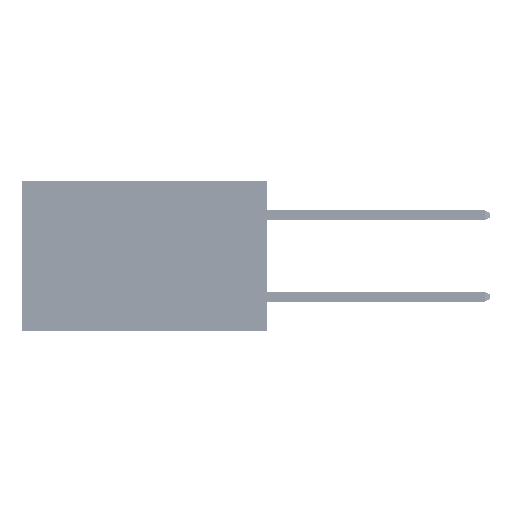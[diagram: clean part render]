
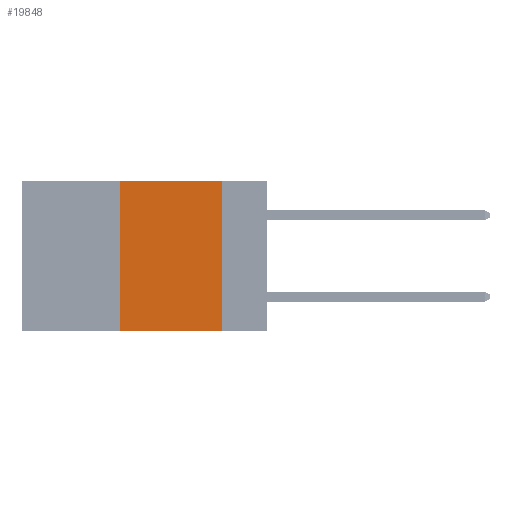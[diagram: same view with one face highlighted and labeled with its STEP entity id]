
A CAD part, left-side view. The second image highlights one B-rep face of the part: STEP entity #19848.
In plain terms, the highlighted planar face has unit normal (-1, 0, 0).
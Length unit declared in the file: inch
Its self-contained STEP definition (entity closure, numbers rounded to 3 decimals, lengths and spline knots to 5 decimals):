
#2881 = DIRECTION ( 'NONE',  ( 0., 0., -1. ) ) ;
#4597 = CARTESIAN_POINT ( 'NONE',  ( 0., 0.11, 0. ) ) ;
#4826 = EDGE_CURVE ( 'NONE', #44555, #21215, #47177, .T. ) ;
#5921 = CARTESIAN_POINT ( 'NONE',  ( 0., 0.6, 0. ) ) ;
#5944 = ORIENTED_EDGE ( 'NONE', *, *, #8604, .T. ) ;
#6163 = EDGE_CURVE ( 'NONE', #28445, #44555, #47015, .T. ) ;
#6891 = CARTESIAN_POINT ( 'NONE',  ( 0., 0.36, 0. ) ) ;
#6893 = ORIENTED_EDGE ( 'NONE', *, *, #46748, .F. ) ;
#8604 = EDGE_CURVE ( 'NONE', #32941, #21215, #31507, .T. ) ;
#9688 = FACE_OUTER_BOUND ( 'NONE', #46534, .T. ) ;
#10430 = VECTOR ( 'NONE', #15764, 39.37008 ) ;
#12742 = CARTESIAN_POINT ( 'NONE',  ( 0., 0.11, 0. ) ) ;
#14281 = ORIENTED_EDGE ( 'NONE', *, *, #4826, .F. ) ;
#14934 = ORIENTED_EDGE ( 'NONE', *, *, #6163, .F. ) ;
#15162 = DIRECTION ( 'NONE',  ( 0., -1., 0. ) ) ;
#15764 = DIRECTION ( 'NONE',  ( 0., -1., 0. ) ) ;
#15938 = CARTESIAN_POINT ( 'NONE',  ( 0., 0.36, -0.37 ) ) ;
#18908 = PLANE ( 'NONE',  #27544 ) ;
#19848 = ADVANCED_FACE ( 'NONE', ( #9688 ), #18908, .F. ) ;
#21215 = VERTEX_POINT ( 'NONE', #35175 ) ;
#23415 = VECTOR ( 'NONE', #42491, 39.37008 ) ;
#25378 = VECTOR ( 'NONE', #15162, 39.37008 ) ;
#26223 = DIRECTION ( 'NONE',  ( 1., 0., 0. ) ) ;
#27544 = AXIS2_PLACEMENT_3D ( 'NONE', #49596, #26223, #2881 ) ;
#28352 = CARTESIAN_POINT ( 'NONE',  ( 0., 0.36, 0. ) ) ;
#28445 = VERTEX_POINT ( 'NONE', #28352 ) ;
#31157 = CARTESIAN_POINT ( 'NONE',  ( 0., 0.6, -0.37 ) ) ;
#31507 = LINE ( 'NONE', #31157, #25378 ) ;
#32941 = VERTEX_POINT ( 'NONE', #15938 ) ;
#35175 = CARTESIAN_POINT ( 'NONE',  ( 0., 0.11, -0.37 ) ) ;
#36833 = VECTOR ( 'NONE', #39683, 39.37008 ) ;
#38700 = LINE ( 'NONE', #6891, #23415 ) ;
#39683 = DIRECTION ( 'NONE',  ( 0., 0., -1. ) ) ;
#42491 = DIRECTION ( 'NONE',  ( 0., 0., 1. ) ) ;
#44555 = VERTEX_POINT ( 'NONE', #4597 ) ;
#46534 = EDGE_LOOP ( 'NONE', ( #14281, #14934, #6893, #5944 ) ) ;
#46748 = EDGE_CURVE ( 'NONE', #32941, #28445, #38700, .T. ) ;
#47015 = LINE ( 'NONE', #5921, #10430 ) ;
#47177 = LINE ( 'NONE', #12742, #36833 ) ;
#49596 = CARTESIAN_POINT ( 'NONE',  ( 0., 0.6, 0. ) ) ;
